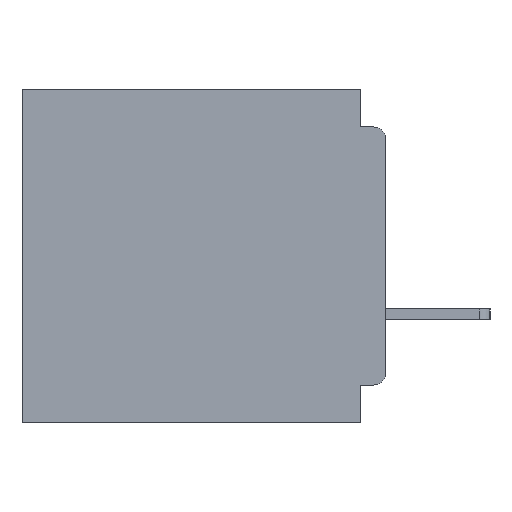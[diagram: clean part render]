
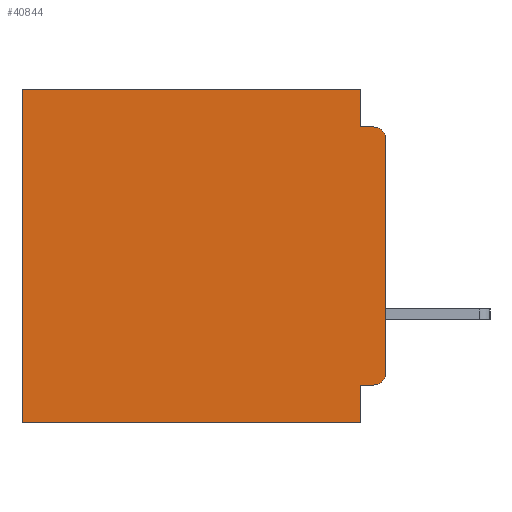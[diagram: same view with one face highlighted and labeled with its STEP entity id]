
A CAD part, left-side view. The second image highlights one B-rep face of the part: STEP entity #40844.
In plain terms, the highlighted planar face has unit normal (-1, 0, 0).
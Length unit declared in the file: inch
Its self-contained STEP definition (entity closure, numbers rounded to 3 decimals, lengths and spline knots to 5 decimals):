
#697 = DIRECTION ( 'NONE',  ( 0., 1., 0. ) ) ;
#894 = ORIENTED_EDGE ( 'NONE', *, *, #13569, .F. ) ;
#1051 = LINE ( 'NONE', #43867, #17519 ) ;
#1429 = VERTEX_POINT ( 'NONE', #5484 ) ;
#1774 = EDGE_CURVE ( 'NONE', #42284, #9409, #43544, .T. ) ;
#2056 = VECTOR ( 'NONE', #36210, 39.37008 ) ;
#2256 = VERTEX_POINT ( 'NONE', #37695 ) ;
#4614 = CARTESIAN_POINT ( 'NONE',  ( 0.3, 0., -0.4 ) ) ;
#5484 = CARTESIAN_POINT ( 'NONE',  ( 0.3, 0.437, 0. ) ) ;
#5584 = EDGE_CURVE ( 'NONE', #35285, #9409, #11430, .T. ) ;
#5770 = DIRECTION ( 'NONE',  ( 0., 1., 0. ) ) ;
#5787 = CARTESIAN_POINT ( 'NONE',  ( 0.3, 0., -0.34 ) ) ;
#7094 = DIRECTION ( 'NONE',  ( 0., 0., -1. ) ) ;
#8027 = LINE ( 'NONE', #17535, #43842 ) ;
#8148 = DIRECTION ( 'NONE',  ( 0., 0., -1. ) ) ;
#8625 = AXIS2_PLACEMENT_3D ( 'NONE', #21491, #21408, #36007 ) ;
#9409 = VERTEX_POINT ( 'NONE', #38737 ) ;
#9745 = CARTESIAN_POINT ( 'NONE',  ( 0.3, 0.031, 0. ) ) ;
#10137 = EDGE_LOOP ( 'NONE', ( #19404, #23765, #43187, #38436, #24379, #11316, #35339, #16273, #894, #13556 ) ) ;
#10720 = AXIS2_PLACEMENT_3D ( 'NONE', #32629, #11738, #36120 ) ;
#10877 = EDGE_CURVE ( 'NONE', #18192, #38222, #28577, .T. ) ;
#11316 = ORIENTED_EDGE ( 'NONE', *, *, #41730, .T. ) ;
#11430 = LINE ( 'NONE', #33042, #2056 ) ;
#11738 = DIRECTION ( 'NONE',  ( -1., 0., 0. ) ) ;
#12532 = LINE ( 'NONE', #21698, #29969 ) ;
#13556 = ORIENTED_EDGE ( 'NONE', *, *, #21444, .T. ) ;
#13569 = EDGE_CURVE ( 'NONE', #2256, #23228, #12532, .T. ) ;
#14122 = EDGE_CURVE ( 'NONE', #23228, #18192, #8027, .T. ) ;
#16067 = LINE ( 'NONE', #43138, #24226 ) ;
#16273 = ORIENTED_EDGE ( 'NONE', *, *, #14122, .F. ) ;
#17519 = VECTOR ( 'NONE', #5770, 39.37008 ) ;
#17535 = CARTESIAN_POINT ( 'NONE',  ( 0.3, 0.031, -0.4 ) ) ;
#17882 = DIRECTION ( 'NONE',  ( 0., 1., 0. ) ) ;
#18192 = VERTEX_POINT ( 'NONE', #23629 ) ;
#18336 = DIRECTION ( 'NONE',  ( 1., 0., 0. ) ) ;
#18353 = FACE_OUTER_BOUND ( 'NONE', #10137, .T. ) ;
#18976 = DIRECTION ( 'NONE',  ( 0., 0., -1. ) ) ;
#19404 = ORIENTED_EDGE ( 'NONE', *, *, #24363, .F. ) ;
#21119 = EDGE_CURVE ( 'NONE', #43479, #35285, #27884, .T. ) ;
#21408 = DIRECTION ( 'NONE',  ( -1., 0., 0. ) ) ;
#21444 = EDGE_CURVE ( 'NONE', #2256, #35093, #22951, .T. ) ;
#21491 = CARTESIAN_POINT ( 'NONE',  ( 0.3, 0.015, -0.06 ) ) ;
#21698 = CARTESIAN_POINT ( 'NONE',  ( 0.3, 0., -0.355 ) ) ;
#22498 = CARTESIAN_POINT ( 'NONE',  ( 0.3, 0.031, 0. ) ) ;
#22951 = CIRCLE ( 'NONE', #10720, 0.015 ) ;
#23228 = VERTEX_POINT ( 'NONE', #24046 ) ;
#23629 = CARTESIAN_POINT ( 'NONE',  ( 0.3, 0.031, -0.4 ) ) ;
#23765 = ORIENTED_EDGE ( 'NONE', *, *, #1774, .T. ) ;
#24046 = CARTESIAN_POINT ( 'NONE',  ( 0.3, 0.031, -0.355 ) ) ;
#24226 = VECTOR ( 'NONE', #18976, 39.37008 ) ;
#24363 = EDGE_CURVE ( 'NONE', #42284, #35093, #28162, .T. ) ;
#24379 = ORIENTED_EDGE ( 'NONE', *, *, #43603, .T. ) ;
#24801 = AXIS2_PLACEMENT_3D ( 'NONE', #39085, #18336, #42507 ) ;
#27508 = VECTOR ( 'NONE', #17882, 39.37008 ) ;
#27884 = LINE ( 'NONE', #9745, #36070 ) ;
#28162 = LINE ( 'NONE', #4614, #37383 ) ;
#28233 = CARTESIAN_POINT ( 'NONE',  ( 0.3, 0., -0.4 ) ) ;
#28577 = LINE ( 'NONE', #28233, #27508 ) ;
#28827 = CARTESIAN_POINT ( 'NONE',  ( 0.3, 0., -0.06 ) ) ;
#29969 = VECTOR ( 'NONE', #697, 39.37008 ) ;
#30685 = DIRECTION ( 'NONE',  ( 0., 0., -1. ) ) ;
#32196 = PLANE ( 'NONE',  #24801 ) ;
#32629 = CARTESIAN_POINT ( 'NONE',  ( 0.3, 0.015, -0.34 ) ) ;
#33042 = CARTESIAN_POINT ( 'NONE',  ( 0.3, 0., -0.045 ) ) ;
#35093 = VERTEX_POINT ( 'NONE', #5787 ) ;
#35285 = VERTEX_POINT ( 'NONE', #38249 ) ;
#35310 = CARTESIAN_POINT ( 'NONE',  ( 0.3, 0.437, -0.4 ) ) ;
#35339 = ORIENTED_EDGE ( 'NONE', *, *, #10877, .F. ) ;
#36007 = DIRECTION ( 'NONE',  ( 0., 0., -1. ) ) ;
#36070 = VECTOR ( 'NONE', #30685, 39.37008 ) ;
#36120 = DIRECTION ( 'NONE',  ( 0., 0., -1. ) ) ;
#36210 = DIRECTION ( 'NONE',  ( 0., -1., 0. ) ) ;
#37383 = VECTOR ( 'NONE', #8148, 39.37008 ) ;
#37695 = CARTESIAN_POINT ( 'NONE',  ( 0.3, 0.015, -0.355 ) ) ;
#38222 = VERTEX_POINT ( 'NONE', #35310 ) ;
#38249 = CARTESIAN_POINT ( 'NONE',  ( 0.3, 0.031, -0.045 ) ) ;
#38436 = ORIENTED_EDGE ( 'NONE', *, *, #21119, .F. ) ;
#38737 = CARTESIAN_POINT ( 'NONE',  ( 0.3, 0.015, -0.045 ) ) ;
#39085 = CARTESIAN_POINT ( 'NONE',  ( 0.3, 0., -0.4 ) ) ;
#40844 = ADVANCED_FACE ( 'NONE', ( #18353 ), #32196, .F. ) ;
#41730 = EDGE_CURVE ( 'NONE', #1429, #38222, #16067, .T. ) ;
#42284 = VERTEX_POINT ( 'NONE', #28827 ) ;
#42507 = DIRECTION ( 'NONE',  ( 0., 0., -1. ) ) ;
#43138 = CARTESIAN_POINT ( 'NONE',  ( 0.3, 0.437, -0.4 ) ) ;
#43187 = ORIENTED_EDGE ( 'NONE', *, *, #5584, .F. ) ;
#43479 = VERTEX_POINT ( 'NONE', #22498 ) ;
#43544 = CIRCLE ( 'NONE', #8625, 0.015 ) ;
#43603 = EDGE_CURVE ( 'NONE', #43479, #1429, #1051, .T. ) ;
#43842 = VECTOR ( 'NONE', #7094, 39.37008 ) ;
#43867 = CARTESIAN_POINT ( 'NONE',  ( 0.3, 0., 0. ) ) ;
